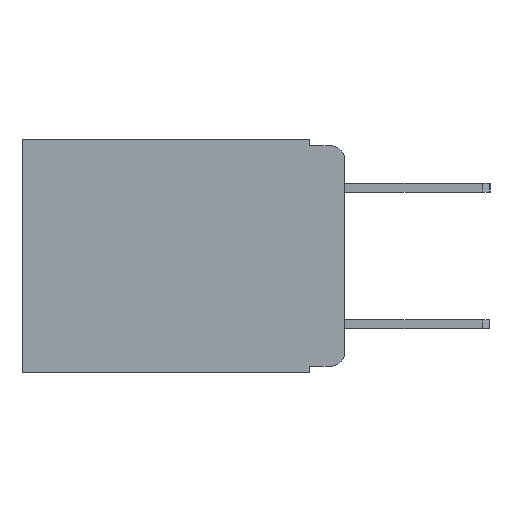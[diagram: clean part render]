
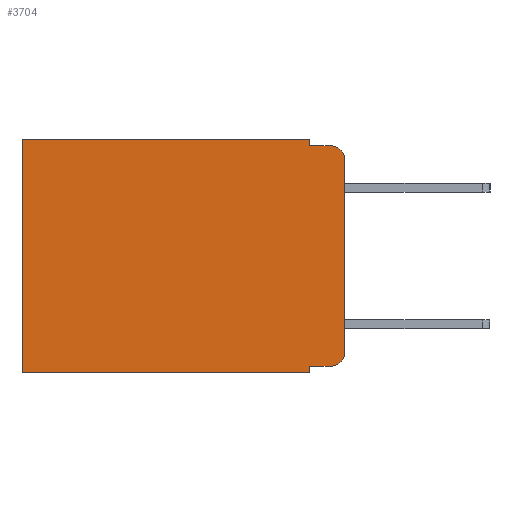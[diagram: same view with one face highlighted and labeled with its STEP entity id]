
A CAD part, left-side view. The second image highlights one B-rep face of the part: STEP entity #3704.
In plain terms, the highlighted planar face has unit normal (-1, 0, 0).
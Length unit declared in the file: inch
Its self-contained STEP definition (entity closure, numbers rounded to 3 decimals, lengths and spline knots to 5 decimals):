
#137 = DIRECTION ( 'NONE',  ( -1., 0., 0. ) ) ;
#143 = AXIS2_PLACEMENT_3D ( 'NONE', #19501, #10749, #1364 ) ;
#272 = DIRECTION ( 'NONE',  ( 0., 0., -1. ) ) ;
#306 = LINE ( 'NONE', #15214, #15826 ) ;
#369 = VERTEX_POINT ( 'NONE', #3206 ) ;
#383 = EDGE_CURVE ( 'NONE', #8585, #369, #15987, .T. ) ;
#396 = VECTOR ( 'NONE', #9424, 39.37008 ) ;
#411 = CARTESIAN_POINT ( 'NONE',  ( 0.298, 0.02, -0.01 ) ) ;
#828 = CARTESIAN_POINT ( 'NONE',  ( 0.298, 0., -0.03 ) ) ;
#900 = VECTOR ( 'NONE', #10526, 39.37008 ) ;
#954 = EDGE_CURVE ( 'NONE', #10706, #5662, #14119, .T. ) ;
#1322 = CARTESIAN_POINT ( 'NONE',  ( 0.298, 0.051, -0.333 ) ) ;
#1364 = DIRECTION ( 'NONE',  ( 0., 0., -1. ) ) ;
#1488 = ORIENTED_EDGE ( 'NONE', *, *, #18722, .T. ) ;
#1509 = VERTEX_POINT ( 'NONE', #7003 ) ;
#1947 = CARTESIAN_POINT ( 'NONE',  ( 0.298, 0., 0. ) ) ;
#2133 = ORIENTED_EDGE ( 'NONE', *, *, #383, .F. ) ;
#2154 = ORIENTED_EDGE ( 'NONE', *, *, #17191, .T. ) ;
#2532 = ORIENTED_EDGE ( 'NONE', *, *, #17400, .F. ) ;
#2819 = DIRECTION ( 'NONE',  ( 1., 0., 0. ) ) ;
#2827 = ORIENTED_EDGE ( 'NONE', *, *, #17874, .T. ) ;
#2844 = CIRCLE ( 'NONE', #143, 0.02 ) ;
#2881 = ORIENTED_EDGE ( 'NONE', *, *, #9463, .F. ) ;
#2958 = DIRECTION ( 'NONE',  ( 0., -1., 0. ) ) ;
#3206 = CARTESIAN_POINT ( 'NONE',  ( 0.298, 0.051, -0.343 ) ) ;
#3704 = ADVANCED_FACE ( 'NONE', ( #4864 ), #5857, .F. ) ;
#3770 = ORIENTED_EDGE ( 'NONE', *, *, #16441, .T. ) ;
#4062 = LINE ( 'NONE', #1947, #10420 ) ;
#4864 = FACE_OUTER_BOUND ( 'NONE', #18948, .T. ) ;
#5037 = CARTESIAN_POINT ( 'NONE',  ( 0.298, 0.051, -0.01 ) ) ;
#5083 = LINE ( 'NONE', #1322, #16739 ) ;
#5089 = VERTEX_POINT ( 'NONE', #12513 ) ;
#5250 = VECTOR ( 'NONE', #272, 39.37008 ) ;
#5662 = VERTEX_POINT ( 'NONE', #411 ) ;
#5857 = PLANE ( 'NONE',  #17618 ) ;
#6267 = EDGE_CURVE ( 'NONE', #16329, #5089, #4062, .T. ) ;
#6407 = DIRECTION ( 'NONE',  ( 0., -1., 0. ) ) ;
#6542 = DIRECTION ( 'NONE',  ( 0., 0., -1. ) ) ;
#7003 = CARTESIAN_POINT ( 'NONE',  ( 0.298, 0.473, 0. ) ) ;
#7231 = CARTESIAN_POINT ( 'NONE',  ( 0.298, 0.051, 0. ) ) ;
#8044 = VECTOR ( 'NONE', #6542, 39.37008 ) ;
#8154 = CARTESIAN_POINT ( 'NONE',  ( 0.298, 0.051, 0. ) ) ;
#8585 = VERTEX_POINT ( 'NONE', #8968 ) ;
#8968 = CARTESIAN_POINT ( 'NONE',  ( 0.298, 0.051, -0.333 ) ) ;
#9424 = DIRECTION ( 'NONE',  ( 0., 1., 0. ) ) ;
#9463 = EDGE_CURVE ( 'NONE', #369, #9918, #13400, .T. ) ;
#9693 = CARTESIAN_POINT ( 'NONE',  ( 0.298, 0.02, -0.03 ) ) ;
#9918 = VERTEX_POINT ( 'NONE', #17941 ) ;
#10108 = VECTOR ( 'NONE', #6407, 39.37008 ) ;
#10420 = VECTOR ( 'NONE', #15708, 39.37008 ) ;
#10526 = DIRECTION ( 'NONE',  ( 0., 0., -1. ) ) ;
#10630 = ORIENTED_EDGE ( 'NONE', *, *, #954, .F. ) ;
#10706 = VERTEX_POINT ( 'NONE', #19151 ) ;
#10741 = ORIENTED_EDGE ( 'NONE', *, *, #6267, .F. ) ;
#10749 = DIRECTION ( 'NONE',  ( -1., 0., 0. ) ) ;
#11184 = DIRECTION ( 'NONE',  ( 0., 0., -1. ) ) ;
#11420 = ORIENTED_EDGE ( 'NONE', *, *, #17211, .T. ) ;
#11568 = VERTEX_POINT ( 'NONE', #13521 ) ;
#12226 = DIRECTION ( 'NONE',  ( 0., 1., 0. ) ) ;
#12513 = CARTESIAN_POINT ( 'NONE',  ( 0.298, 0., -0.313 ) ) ;
#12576 = LINE ( 'NONE', #8154, #8044 ) ;
#13400 = LINE ( 'NONE', #18289, #396 ) ;
#13439 = AXIS2_PLACEMENT_3D ( 'NONE', #9693, #137, #11184 ) ;
#13521 = CARTESIAN_POINT ( 'NONE',  ( 0.298, 0.051, 0. ) ) ;
#13635 = DIRECTION ( 'NONE',  ( 0., 0., -1. ) ) ;
#14119 = LINE ( 'NONE', #5037, #10108 ) ;
#15214 = CARTESIAN_POINT ( 'NONE',  ( 0.298, 0., 0. ) ) ;
#15708 = DIRECTION ( 'NONE',  ( 0., 0., -1. ) ) ;
#15826 = VECTOR ( 'NONE', #12226, 39.37008 ) ;
#15849 = VERTEX_POINT ( 'NONE', #16335 ) ;
#15987 = LINE ( 'NONE', #7231, #5250 ) ;
#16329 = VERTEX_POINT ( 'NONE', #828 ) ;
#16335 = CARTESIAN_POINT ( 'NONE',  ( 0.298, 0.02, -0.333 ) ) ;
#16441 = EDGE_CURVE ( 'NONE', #1509, #9918, #17223, .T. ) ;
#16739 = VECTOR ( 'NONE', #2958, 39.37008 ) ;
#17191 = EDGE_CURVE ( 'NONE', #8585, #15849, #5083, .T. ) ;
#17211 = EDGE_CURVE ( 'NONE', #11568, #1509, #306, .T. ) ;
#17223 = LINE ( 'NONE', #19297, #900 ) ;
#17400 = EDGE_CURVE ( 'NONE', #11568, #10706, #12576, .T. ) ;
#17618 = AXIS2_PLACEMENT_3D ( 'NONE', #19340, #2819, #13635 ) ;
#17874 = EDGE_CURVE ( 'NONE', #15849, #5089, #2844, .T. ) ;
#17941 = CARTESIAN_POINT ( 'NONE',  ( 0.298, 0.473, -0.343 ) ) ;
#18289 = CARTESIAN_POINT ( 'NONE',  ( 0.298, 0., -0.343 ) ) ;
#18722 = EDGE_CURVE ( 'NONE', #16329, #5662, #19738, .T. ) ;
#18948 = EDGE_LOOP ( 'NONE', ( #10741, #1488, #10630, #2532, #11420, #3770, #2881, #2133, #2154, #2827 ) ) ;
#19151 = CARTESIAN_POINT ( 'NONE',  ( 0.298, 0.051, -0.01 ) ) ;
#19297 = CARTESIAN_POINT ( 'NONE',  ( 0.298, 0.473, 0. ) ) ;
#19340 = CARTESIAN_POINT ( 'NONE',  ( 0.298, 0., 0. ) ) ;
#19501 = CARTESIAN_POINT ( 'NONE',  ( 0.298, 0.02, -0.313 ) ) ;
#19738 = CIRCLE ( 'NONE', #13439, 0.02 ) ;
